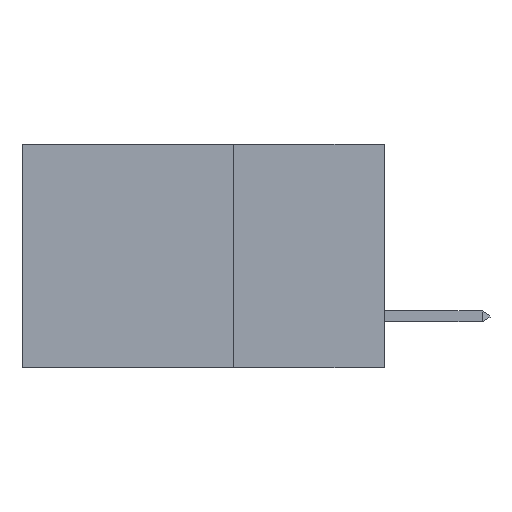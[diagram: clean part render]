
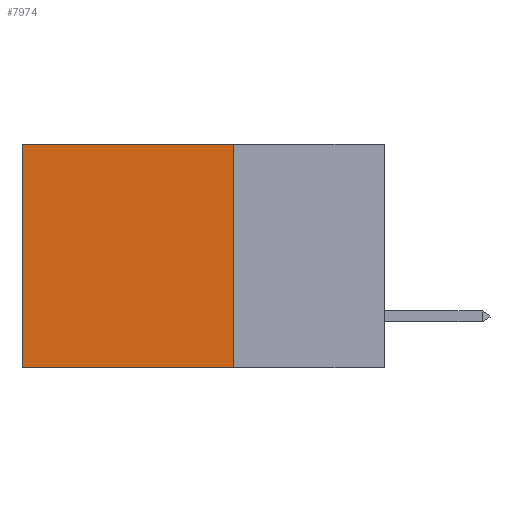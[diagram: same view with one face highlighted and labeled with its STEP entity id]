
A CAD part, left-side view. The second image highlights one B-rep face of the part: STEP entity #7974.
In plain terms, the highlighted planar face has unit normal (-1, 0, 0).
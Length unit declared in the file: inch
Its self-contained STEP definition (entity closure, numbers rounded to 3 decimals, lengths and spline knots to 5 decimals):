
#161 = VERTEX_POINT ( 'NONE', #9213 ) ;
#738 = CARTESIAN_POINT ( 'NONE',  ( 0.2875, 0.25, 0. ) ) ;
#983 = EDGE_CURVE ( 'NONE', #5297, #2021, #4464, .T. ) ;
#1695 = ORIENTED_EDGE ( 'NONE', *, *, #3364, .F. ) ;
#2021 = VERTEX_POINT ( 'NONE', #5245 ) ;
#2049 = PLANE ( 'NONE',  #3956 ) ;
#2100 = DIRECTION ( 'NONE',  ( 1., 0., 0. ) ) ;
#2795 = EDGE_LOOP ( 'NONE', ( #8290, #1695, #11117, #10393 ) ) ;
#3364 = EDGE_CURVE ( 'NONE', #2021, #6827, #7179, .T. ) ;
#3956 = AXIS2_PLACEMENT_3D ( 'NONE', #7072, #2100, #8938 ) ;
#3962 = FACE_OUTER_BOUND ( 'NONE', #2795, .T. ) ;
#4141 = VECTOR ( 'NONE', #8561, 39.37008 ) ;
#4464 = LINE ( 'NONE', #738, #4141 ) ;
#4559 = VECTOR ( 'NONE', #6364, 39.37008 ) ;
#5109 = VECTOR ( 'NONE', #12458, 39.37008 ) ;
#5245 = CARTESIAN_POINT ( 'NONE',  ( 0.2875, 0.25, -0.37 ) ) ;
#5281 = EDGE_CURVE ( 'NONE', #5297, #161, #5286, .T. ) ;
#5286 = LINE ( 'NONE', #11248, #10064 ) ;
#5297 = VERTEX_POINT ( 'NONE', #9398 ) ;
#5573 = EDGE_CURVE ( 'NONE', #161, #6827, #7700, .T. ) ;
#5949 = CARTESIAN_POINT ( 'NONE',  ( 0.2875, 0.6, 0. ) ) ;
#6364 = DIRECTION ( 'NONE',  ( 0., 1., 0. ) ) ;
#6827 = VERTEX_POINT ( 'NONE', #10365 ) ;
#7072 = CARTESIAN_POINT ( 'NONE',  ( 0.2875, 0.25, 0. ) ) ;
#7179 = LINE ( 'NONE', #10158, #4559 ) ;
#7700 = LINE ( 'NONE', #5949, #5109 ) ;
#7974 = ADVANCED_FACE ( 'NONE', ( #3962 ), #2049, .F. ) ;
#8290 = ORIENTED_EDGE ( 'NONE', *, *, #5573, .T. ) ;
#8561 = DIRECTION ( 'NONE',  ( 0., 0., -1. ) ) ;
#8938 = DIRECTION ( 'NONE',  ( 0., 0., -1. ) ) ;
#9213 = CARTESIAN_POINT ( 'NONE',  ( 0.2875, 0.6, 0. ) ) ;
#9398 = CARTESIAN_POINT ( 'NONE',  ( 0.2875, 0.25, 0. ) ) ;
#10064 = VECTOR ( 'NONE', #10351, 39.37008 ) ;
#10158 = CARTESIAN_POINT ( 'NONE',  ( 0.2875, 0.25, -0.37 ) ) ;
#10351 = DIRECTION ( 'NONE',  ( 0., 1., 0. ) ) ;
#10365 = CARTESIAN_POINT ( 'NONE',  ( 0.2875, 0.6, -0.37 ) ) ;
#10393 = ORIENTED_EDGE ( 'NONE', *, *, #5281, .T. ) ;
#11117 = ORIENTED_EDGE ( 'NONE', *, *, #983, .F. ) ;
#11248 = CARTESIAN_POINT ( 'NONE',  ( 0.2875, 0.25, 0. ) ) ;
#12458 = DIRECTION ( 'NONE',  ( 0., 0., -1. ) ) ;
